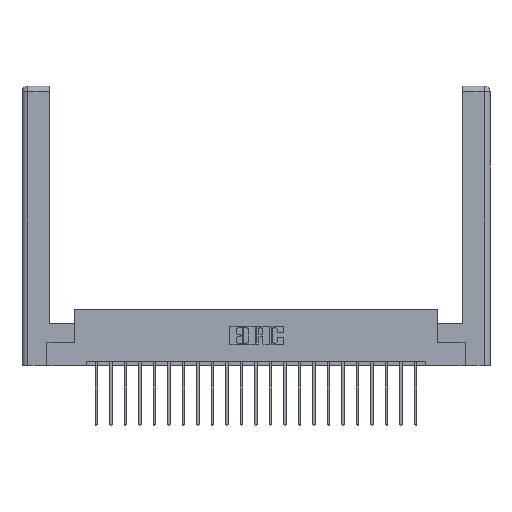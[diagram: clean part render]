
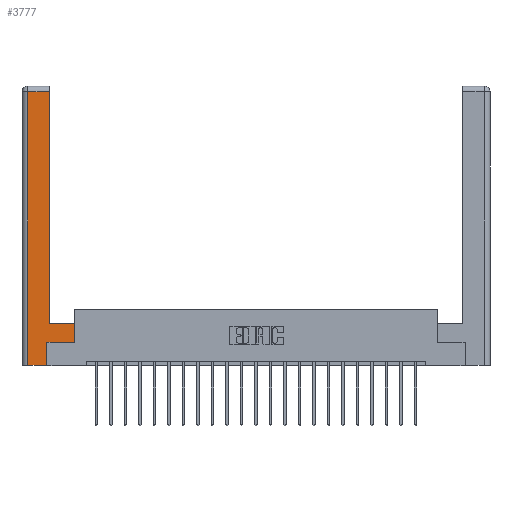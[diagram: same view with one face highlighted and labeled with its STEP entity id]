
A CAD part, top view. The second image highlights one B-rep face of the part: STEP entity #3777.
In plain terms, the highlighted planar face has unit normal (0, 0, 1).
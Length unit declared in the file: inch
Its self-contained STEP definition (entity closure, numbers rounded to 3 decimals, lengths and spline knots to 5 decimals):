
#242 = VECTOR ( 'NONE', #12744, 39.37008 ) ;
#904 = CARTESIAN_POINT ( 'NONE',  ( 0.265, 0., 0. ) ) ;
#1103 = ORIENTED_EDGE ( 'NONE', *, *, #2774, .T. ) ;
#1366 = LINE ( 'NONE', #22736, #14959 ) ;
#1567 = DIRECTION ( 'NONE',  ( 0., 1., 0. ) ) ;
#1623 = ORIENTED_EDGE ( 'NONE', *, *, #20002, .T. ) ;
#2011 = DIRECTION ( 'NONE',  ( 0., 1., 0. ) ) ;
#2577 = VERTEX_POINT ( 'NONE', #21628 ) ;
#2584 = VECTOR ( 'NONE', #18210, 39.37008 ) ;
#2774 = EDGE_CURVE ( 'NONE', #22013, #2577, #4084, .T. ) ;
#2887 = VERTEX_POINT ( 'NONE', #5979 ) ;
#3076 = DIRECTION ( 'NONE',  ( -1., 0., 0. ) ) ;
#3316 = CARTESIAN_POINT ( 'NONE',  ( 0.295, 0.45, 0. ) ) ;
#3777 = ADVANCED_FACE ( 'NONE', ( #22436 ), #22961, .F. ) ;
#3867 = VERTEX_POINT ( 'NONE', #14900 ) ;
#4084 = LINE ( 'NONE', #17958, #19094 ) ;
#5188 = CARTESIAN_POINT ( 'NONE',  ( 0., 0., 0. ) ) ;
#5202 = CARTESIAN_POINT ( 'NONE',  ( 0.565, 0.45, 0. ) ) ;
#5381 = LINE ( 'NONE', #13819, #14277 ) ;
#5610 = AXIS2_PLACEMENT_3D ( 'NONE', #5188, #17950, #19487 ) ;
#5777 = CARTESIAN_POINT ( 'NONE',  ( 0.565, 0.245, 0. ) ) ;
#5979 = CARTESIAN_POINT ( 'NONE',  ( 0.565, 0.245, 0. ) ) ;
#6359 = DIRECTION ( 'NONE',  ( -1., 0., 0. ) ) ;
#6457 = EDGE_CURVE ( 'NONE', #3867, #22013, #5381, .T. ) ;
#6463 = LINE ( 'NONE', #5202, #17869 ) ;
#6473 = CARTESIAN_POINT ( 'NONE',  ( 0.0615, 0., 0. ) ) ;
#6778 = EDGE_CURVE ( 'NONE', #13130, #2887, #17648, .T. ) ;
#7381 = VERTEX_POINT ( 'NONE', #20022 ) ;
#10216 = ORIENTED_EDGE ( 'NONE', *, *, #21429, .T. ) ;
#10279 = EDGE_CURVE ( 'NONE', #2887, #3867, #6463, .T. ) ;
#10739 = CARTESIAN_POINT ( 'NONE',  ( 0.265, 0., 0. ) ) ;
#12262 = VECTOR ( 'NONE', #15092, 39.37008 ) ;
#12744 = DIRECTION ( 'NONE',  ( 0., -1., 0. ) ) ;
#13128 = ORIENTED_EDGE ( 'NONE', *, *, #6778, .T. ) ;
#13130 = VERTEX_POINT ( 'NONE', #20012 ) ;
#13819 = CARTESIAN_POINT ( 'NONE',  ( 0.295, 0.45, 0. ) ) ;
#13949 = EDGE_LOOP ( 'NONE', ( #1103, #20403, #10216, #1623, #17271, #13128, #19309, #22744 ) ) ;
#14136 = DIRECTION ( 'NONE',  ( 0., 1., 0. ) ) ;
#14277 = VECTOR ( 'NONE', #3076, 39.37008 ) ;
#14502 = CARTESIAN_POINT ( 'NONE',  ( 0.0615, 0., 0. ) ) ;
#14900 = CARTESIAN_POINT ( 'NONE',  ( 0.565, 0.45, 0. ) ) ;
#14959 = VECTOR ( 'NONE', #1567, 39.37008 ) ;
#15092 = DIRECTION ( 'NONE',  ( 1., 0., 0. ) ) ;
#15321 = VERTEX_POINT ( 'NONE', #10739 ) ;
#15847 = VERTEX_POINT ( 'NONE', #6473 ) ;
#16912 = LINE ( 'NONE', #18781, #22166 ) ;
#17271 = ORIENTED_EDGE ( 'NONE', *, *, #22007, .T. ) ;
#17648 = LINE ( 'NONE', #5777, #2584 ) ;
#17869 = VECTOR ( 'NONE', #14136, 39.37008 ) ;
#17950 = DIRECTION ( 'NONE',  ( 0., 0., -1. ) ) ;
#17958 = CARTESIAN_POINT ( 'NONE',  ( 0.295, 3., 0. ) ) ;
#18210 = DIRECTION ( 'NONE',  ( 1., 0., 0. ) ) ;
#18781 = CARTESIAN_POINT ( 'NONE',  ( 0.0615, 2.94, 0. ) ) ;
#19094 = VECTOR ( 'NONE', #2011, 39.37008 ) ;
#19309 = ORIENTED_EDGE ( 'NONE', *, *, #10279, .T. ) ;
#19487 = DIRECTION ( 'NONE',  ( -1., 0., 0. ) ) ;
#20002 = EDGE_CURVE ( 'NONE', #15847, #15321, #21665, .T. ) ;
#20012 = CARTESIAN_POINT ( 'NONE',  ( 0.265, 0.245, 0. ) ) ;
#20022 = CARTESIAN_POINT ( 'NONE',  ( 0.0615, 2.94, 0. ) ) ;
#20403 = ORIENTED_EDGE ( 'NONE', *, *, #21063, .T. ) ;
#21063 = EDGE_CURVE ( 'NONE', #2577, #7381, #16912, .T. ) ;
#21429 = EDGE_CURVE ( 'NONE', #7381, #15847, #22413, .T. ) ;
#21628 = CARTESIAN_POINT ( 'NONE',  ( 0.295, 2.94, 0. ) ) ;
#21665 = LINE ( 'NONE', #904, #12262 ) ;
#22007 = EDGE_CURVE ( 'NONE', #15321, #13130, #1366, .T. ) ;
#22013 = VERTEX_POINT ( 'NONE', #3316 ) ;
#22166 = VECTOR ( 'NONE', #6359, 39.37008 ) ;
#22413 = LINE ( 'NONE', #14502, #242 ) ;
#22436 = FACE_OUTER_BOUND ( 'NONE', #13949, .T. ) ;
#22736 = CARTESIAN_POINT ( 'NONE',  ( 0.265, 0.245, 0. ) ) ;
#22744 = ORIENTED_EDGE ( 'NONE', *, *, #6457, .T. ) ;
#22961 = PLANE ( 'NONE',  #5610 ) ;
